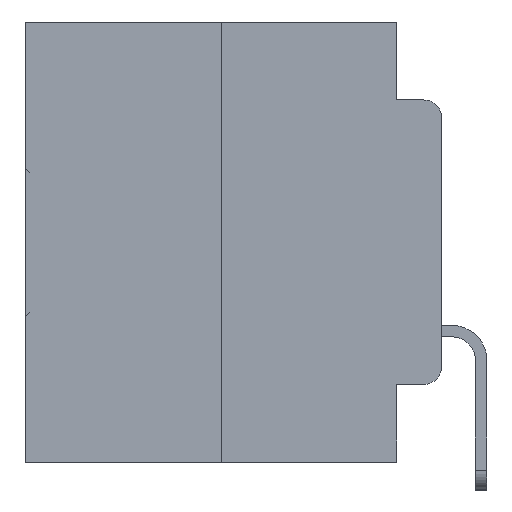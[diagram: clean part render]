
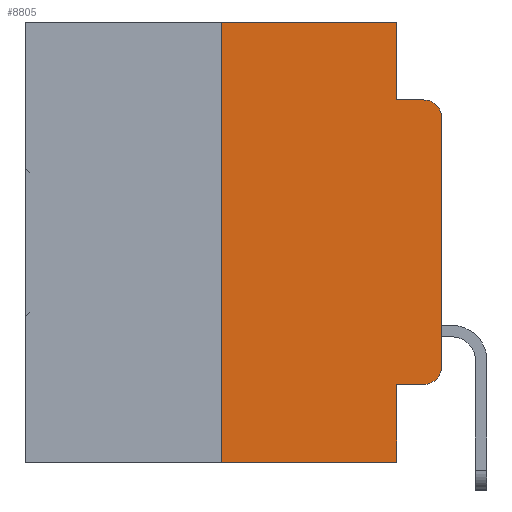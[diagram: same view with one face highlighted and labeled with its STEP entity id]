
A CAD part, left-side view. The second image highlights one B-rep face of the part: STEP entity #8805.
In plain terms, the highlighted planar face has unit normal (-1, 0, 0).
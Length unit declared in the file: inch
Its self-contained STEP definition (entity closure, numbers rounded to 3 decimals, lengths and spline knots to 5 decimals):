
#32 = VECTOR ( 'NONE', #20731, 39.37008 ) ;
#273 = VERTEX_POINT ( 'NONE', #22928 ) ;
#1001 = DIRECTION ( 'NONE',  ( 1., 0., 0. ) ) ;
#1957 = CARTESIAN_POINT ( 'NONE',  ( 0., 0.02, -0.3915 ) ) ;
#2074 = CIRCLE ( 'NONE', #19417, 0.02 ) ;
#2087 = CARTESIAN_POINT ( 'NONE',  ( 0., 0.051, -0.5 ) ) ;
#2820 = DIRECTION ( 'NONE',  ( 0., -1., 0. ) ) ;
#3381 = VERTEX_POINT ( 'NONE', #23086 ) ;
#3534 = CARTESIAN_POINT ( 'NONE',  ( 0., 0.02, -0.4115 ) ) ;
#4001 = VERTEX_POINT ( 'NONE', #4474 ) ;
#4007 = ORIENTED_EDGE ( 'NONE', *, *, #25820, .F. ) ;
#4474 = CARTESIAN_POINT ( 'NONE',  ( 0., 0., -0.3915 ) ) ;
#4575 = DIRECTION ( 'NONE',  ( 0., 0., -1. ) ) ;
#4964 = VECTOR ( 'NONE', #23433, 39.37008 ) ;
#5025 = DIRECTION ( 'NONE',  ( 0., 0., -1. ) ) ;
#6076 = DIRECTION ( 'NONE',  ( 0., 0., -1. ) ) ;
#6149 = AXIS2_PLACEMENT_3D ( 'NONE', #24992, #1001, #18398 ) ;
#6164 = VERTEX_POINT ( 'NONE', #16331 ) ;
#6303 = CARTESIAN_POINT ( 'NONE',  ( 0., 0.473, -0.5 ) ) ;
#6567 = LINE ( 'NONE', #24514, #30537 ) ;
#6976 = EDGE_CURVE ( 'NONE', #12876, #9901, #23310, .T. ) ;
#6996 = LINE ( 'NONE', #6303, #32 ) ;
#7474 = CARTESIAN_POINT ( 'NONE',  ( 0., 0.051, 0. ) ) ;
#7757 = EDGE_CURVE ( 'NONE', #9901, #273, #17381, .T. ) ;
#7878 = AXIS2_PLACEMENT_3D ( 'NONE', #1957, #19216, #4575 ) ;
#8114 = CARTESIAN_POINT ( 'NONE',  ( 0., 0.051, -0.0885 ) ) ;
#8692 = EDGE_CURVE ( 'NONE', #4001, #18711, #6567, .T. ) ;
#8805 = ADVANCED_FACE ( 'NONE', ( #26359 ), #29466, .F. ) ;
#9328 = EDGE_CURVE ( 'NONE', #20062, #3381, #14427, .T. ) ;
#9425 = CARTESIAN_POINT ( 'NONE',  ( 0., 0.25, 0. ) ) ;
#9901 = VERTEX_POINT ( 'NONE', #22754 ) ;
#10008 = DIRECTION ( 'NONE',  ( 0., 0., -1. ) ) ;
#11734 = EDGE_LOOP ( 'NONE', ( #26220, #17160, #19298, #20705, #22807, #18233, #13519, #4007, #18608, #25202 ) ) ;
#12042 = LINE ( 'NONE', #25748, #30149 ) ;
#12063 = DIRECTION ( 'NONE',  ( 0., -1., 0. ) ) ;
#12100 = CARTESIAN_POINT ( 'NONE',  ( 0., 0.25, -0.5 ) ) ;
#12690 = VERTEX_POINT ( 'NONE', #3534 ) ;
#12876 = VERTEX_POINT ( 'NONE', #12100 ) ;
#13519 = ORIENTED_EDGE ( 'NONE', *, *, #24450, .T. ) ;
#14427 = LINE ( 'NONE', #8114, #19775 ) ;
#15615 = DIRECTION ( 'NONE',  ( 0., 0., 1. ) ) ;
#15789 = CARTESIAN_POINT ( 'NONE',  ( 0., 0.473, 0. ) ) ;
#16331 = CARTESIAN_POINT ( 'NONE',  ( 0., 0.051, -0.4115 ) ) ;
#16683 = VECTOR ( 'NONE', #24772, 39.37008 ) ;
#17160 = ORIENTED_EDGE ( 'NONE', *, *, #19877, .T. ) ;
#17381 = LINE ( 'NONE', #15789, #16683 ) ;
#17636 = EDGE_CURVE ( 'NONE', #12690, #4001, #30097, .T. ) ;
#18233 = ORIENTED_EDGE ( 'NONE', *, *, #6976, .F. ) ;
#18398 = DIRECTION ( 'NONE',  ( 0., 0., -1. ) ) ;
#18608 = ORIENTED_EDGE ( 'NONE', *, *, #19344, .T. ) ;
#18711 = VERTEX_POINT ( 'NONE', #28392 ) ;
#19216 = DIRECTION ( 'NONE',  ( -1., 0., 0. ) ) ;
#19298 = ORIENTED_EDGE ( 'NONE', *, *, #9328, .F. ) ;
#19344 = EDGE_CURVE ( 'NONE', #6164, #12690, #12042, .T. ) ;
#19417 = AXIS2_PLACEMENT_3D ( 'NONE', #22256, #20536, #6076 ) ;
#19775 = VECTOR ( 'NONE', #2820, 39.37008 ) ;
#19877 = EDGE_CURVE ( 'NONE', #18711, #3381, #2074, .T. ) ;
#20062 = VERTEX_POINT ( 'NONE', #27591 ) ;
#20536 = DIRECTION ( 'NONE',  ( -1., 0., 0. ) ) ;
#20705 = ORIENTED_EDGE ( 'NONE', *, *, #30839, .F. ) ;
#20731 = DIRECTION ( 'NONE',  ( 0., -1., 0. ) ) ;
#22256 = CARTESIAN_POINT ( 'NONE',  ( 0., 0.02, -0.1085 ) ) ;
#22754 = CARTESIAN_POINT ( 'NONE',  ( 0., 0.25, 0. ) ) ;
#22807 = ORIENTED_EDGE ( 'NONE', *, *, #7757, .F. ) ;
#22897 = VECTOR ( 'NONE', #5025, 39.37008 ) ;
#22928 = CARTESIAN_POINT ( 'NONE',  ( 0., 0.051, 0. ) ) ;
#23086 = CARTESIAN_POINT ( 'NONE',  ( 0., 0.02, -0.0885 ) ) ;
#23203 = VERTEX_POINT ( 'NONE', #2087 ) ;
#23310 = LINE ( 'NONE', #9425, #4964 ) ;
#23433 = DIRECTION ( 'NONE',  ( 0., 0., 1. ) ) ;
#23585 = LINE ( 'NONE', #26296, #22897 ) ;
#24450 = EDGE_CURVE ( 'NONE', #12876, #23203, #6996, .T. ) ;
#24514 = CARTESIAN_POINT ( 'NONE',  ( 0., 0., 0. ) ) ;
#24772 = DIRECTION ( 'NONE',  ( 0., -1., 0. ) ) ;
#24889 = VECTOR ( 'NONE', #10008, 39.37008 ) ;
#24992 = CARTESIAN_POINT ( 'NONE',  ( 0., 0.473, 0. ) ) ;
#25202 = ORIENTED_EDGE ( 'NONE', *, *, #17636, .T. ) ;
#25748 = CARTESIAN_POINT ( 'NONE',  ( 0., 0.051, -0.4115 ) ) ;
#25820 = EDGE_CURVE ( 'NONE', #6164, #23203, #23585, .T. ) ;
#26220 = ORIENTED_EDGE ( 'NONE', *, *, #8692, .T. ) ;
#26296 = CARTESIAN_POINT ( 'NONE',  ( 0., 0.051, 0. ) ) ;
#26359 = FACE_OUTER_BOUND ( 'NONE', #11734, .T. ) ;
#27591 = CARTESIAN_POINT ( 'NONE',  ( 0., 0.051, -0.0885 ) ) ;
#28392 = CARTESIAN_POINT ( 'NONE',  ( 0., 0., -0.1085 ) ) ;
#29466 = PLANE ( 'NONE',  #6149 ) ;
#30097 = CIRCLE ( 'NONE', #7878, 0.02 ) ;
#30149 = VECTOR ( 'NONE', #12063, 39.37008 ) ;
#30537 = VECTOR ( 'NONE', #15615, 39.37008 ) ;
#30810 = LINE ( 'NONE', #7474, #24889 ) ;
#30839 = EDGE_CURVE ( 'NONE', #273, #20062, #30810, .T. ) ;
